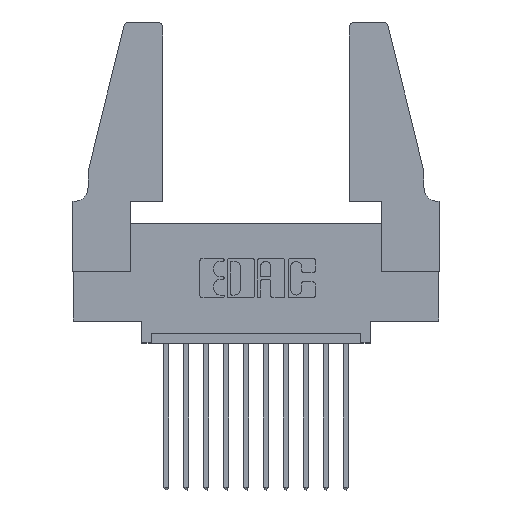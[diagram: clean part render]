
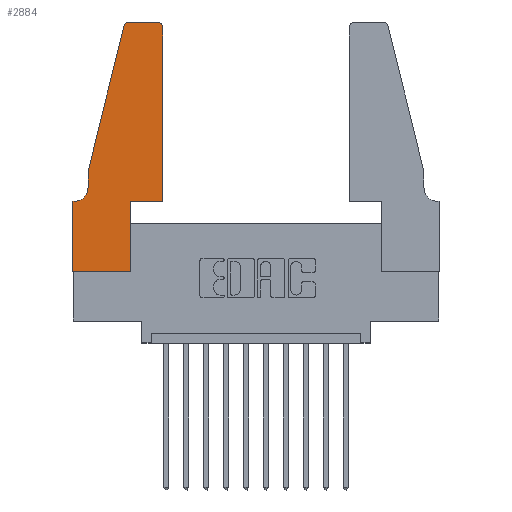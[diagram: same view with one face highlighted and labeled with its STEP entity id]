
A CAD part, top view. The second image highlights one B-rep face of the part: STEP entity #2884.
In plain terms, the highlighted planar face has unit normal (0, 0, 1).
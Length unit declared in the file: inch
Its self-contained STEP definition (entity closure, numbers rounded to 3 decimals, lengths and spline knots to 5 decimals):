
#29 = CARTESIAN_POINT ( 'NONE',  ( 0.2865, 0.35, 0.37 ) ) ;
#145 = LINE ( 'NONE', #1771, #10566 ) ;
#264 = VECTOR ( 'NONE', #11475, 39.37008 ) ;
#322 = AXIS2_PLACEMENT_3D ( 'NONE', #8340, #4215, #11858 ) ;
#350 = EDGE_CURVE ( 'NONE', #7436, #12567, #10413, .T. ) ;
#543 = ORIENTED_EDGE ( 'NONE', *, *, #13548, .T. ) ;
#614 = CARTESIAN_POINT ( 'NONE',  ( 0.2865, 0.35, 0.37 ) ) ;
#729 = LINE ( 'NONE', #6120, #3110 ) ;
#844 = VECTOR ( 'NONE', #7681, 39.37008 ) ;
#951 = VECTOR ( 'NONE', #7058, 39.37008 ) ;
#1074 = EDGE_CURVE ( 'NONE', #11638, #10250, #145, .T. ) ;
#1197 = ORIENTED_EDGE ( 'NONE', *, *, #11548, .T. ) ;
#1418 = VERTEX_POINT ( 'NONE', #29 ) ;
#1538 = VERTEX_POINT ( 'NONE', #4657 ) ;
#1735 = DIRECTION ( 'NONE',  ( 0., 0., -1. ) ) ;
#1771 = CARTESIAN_POINT ( 'NONE',  ( 0., 0., 0.37 ) ) ;
#1780 = LINE ( 'NONE', #6928, #264 ) ;
#2052 = EDGE_LOOP ( 'NONE', ( #7358, #9574, #12502, #6015, #12945, #13895, #11862, #543, #1197, #10156, #3249, #10666 ) ) ;
#2091 = CARTESIAN_POINT ( 'NONE',  ( 0., 0., 0.37 ) ) ;
#2102 = LINE ( 'NONE', #614, #4160 ) ;
#2114 = CIRCLE ( 'NONE', #3457, 0.03 ) ;
#2884 = ADVANCED_FACE ( 'NONE', ( #6073 ), #10430, .T. ) ;
#3110 = VECTOR ( 'NONE', #7028, 39.37008 ) ;
#3249 = ORIENTED_EDGE ( 'NONE', *, *, #4738, .T. ) ;
#3317 = CARTESIAN_POINT ( 'NONE',  ( 0.0755, 0.35, 0.37 ) ) ;
#3360 = VERTEX_POINT ( 'NONE', #12187 ) ;
#3457 = AXIS2_PLACEMENT_3D ( 'NONE', #10304, #4870, #12316 ) ;
#3508 = EDGE_CURVE ( 'NONE', #1418, #3654, #8292, .T. ) ;
#3521 = CARTESIAN_POINT ( 'NONE',  ( 0.284, 1.25, 0.37 ) ) ;
#3654 = VERTEX_POINT ( 'NONE', #13065 ) ;
#3735 = EDGE_CURVE ( 'NONE', #12781, #3360, #6061, .T. ) ;
#3913 = CARTESIAN_POINT ( 'NONE',  ( 0.4505, 0.35, 0.37 ) ) ;
#4008 = DIRECTION ( 'NONE',  ( 1., 0., 0. ) ) ;
#4160 = VECTOR ( 'NONE', #13800, 39.37008 ) ;
#4215 = DIRECTION ( 'NONE',  ( 0., 0., 1. ) ) ;
#4657 = CARTESIAN_POINT ( 'NONE',  ( 0.2865, 0., 0.37 ) ) ;
#4738 = EDGE_CURVE ( 'NONE', #3654, #9921, #729, .T. ) ;
#4870 = DIRECTION ( 'NONE',  ( 0., 0., 1. ) ) ;
#4915 = CARTESIAN_POINT ( 'NONE',  ( 0.0755, 0.5, 0.37 ) ) ;
#5088 = VERTEX_POINT ( 'NONE', #8239 ) ;
#5099 = CARTESIAN_POINT ( 'NONE',  ( 0.4505, 1.22, 0.37 ) ) ;
#5734 = LINE ( 'NONE', #3317, #11729 ) ;
#5951 = DIRECTION ( 'NONE',  ( 0., 0., 1. ) ) ;
#5979 = DIRECTION ( 'NONE',  ( -1., 0., 0. ) ) ;
#6015 = ORIENTED_EDGE ( 'NONE', *, *, #9546, .T. ) ;
#6061 = CIRCLE ( 'NONE', #7648, 0.07 ) ;
#6073 = FACE_OUTER_BOUND ( 'NONE', #2052, .T. ) ;
#6120 = CARTESIAN_POINT ( 'NONE',  ( 0.4505, 0.35, 0.37 ) ) ;
#6133 = AXIS2_PLACEMENT_3D ( 'NONE', #8189, #5951, #6865 ) ;
#6649 = LINE ( 'NONE', #10768, #844 ) ;
#6865 = DIRECTION ( 'NONE',  ( 1., 0., 0. ) ) ;
#6928 = CARTESIAN_POINT ( 'NONE',  ( 0.0755, 0.5, 0.37 ) ) ;
#7028 = DIRECTION ( 'NONE',  ( 0., 1., 0. ) ) ;
#7058 = DIRECTION ( 'NONE',  ( 0., -1., 0. ) ) ;
#7194 = CARTESIAN_POINT ( 'NONE',  ( 0.0055, 0.42, 0.37 ) ) ;
#7358 = ORIENTED_EDGE ( 'NONE', *, *, #350, .T. ) ;
#7436 = VERTEX_POINT ( 'NONE', #7452 ) ;
#7452 = CARTESIAN_POINT ( 'NONE',  ( 0.4205, 1.25, 0.37 ) ) ;
#7487 = CIRCLE ( 'NONE', #6133, 0.03 ) ;
#7648 = AXIS2_PLACEMENT_3D ( 'NONE', #7194, #1735, #12690 ) ;
#7681 = DIRECTION ( 'NONE',  ( 1., 0., 0. ) ) ;
#7960 = LINE ( 'NONE', #4915, #951 ) ;
#8189 = CARTESIAN_POINT ( 'NONE',  ( 0.284, 1.22, 0.37 ) ) ;
#8239 = CARTESIAN_POINT ( 'NONE',  ( 0.0755, 0.5, 0.37 ) ) ;
#8292 = LINE ( 'NONE', #3913, #10675 ) ;
#8305 = CARTESIAN_POINT ( 'NONE',  ( 0.0755, 0.42, 0.37 ) ) ;
#8340 = CARTESIAN_POINT ( 'NONE',  ( 0., 0.35, 0.37 ) ) ;
#8941 = EDGE_CURVE ( 'NONE', #11918, #5088, #1780, .T. ) ;
#9327 = EDGE_CURVE ( 'NONE', #12567, #11918, #7487, .T. ) ;
#9546 = EDGE_CURVE ( 'NONE', #5088, #12781, #7960, .T. ) ;
#9552 = VECTOR ( 'NONE', #5979, 39.37008 ) ;
#9574 = ORIENTED_EDGE ( 'NONE', *, *, #9327, .T. ) ;
#9765 = EDGE_CURVE ( 'NONE', #3360, #11638, #5734, .T. ) ;
#9921 = VERTEX_POINT ( 'NONE', #5099 ) ;
#9983 = CARTESIAN_POINT ( 'NONE',  ( 0.25487, 1.22718, 0.37 ) ) ;
#10156 = ORIENTED_EDGE ( 'NONE', *, *, #3508, .T. ) ;
#10250 = VERTEX_POINT ( 'NONE', #2091 ) ;
#10304 = CARTESIAN_POINT ( 'NONE',  ( 0.4205, 1.22, 0.37 ) ) ;
#10413 = LINE ( 'NONE', #12434, #9552 ) ;
#10430 = PLANE ( 'NONE',  #322 ) ;
#10566 = VECTOR ( 'NONE', #11637, 39.37008 ) ;
#10666 = ORIENTED_EDGE ( 'NONE', *, *, #11415, .T. ) ;
#10675 = VECTOR ( 'NONE', #4008, 39.37008 ) ;
#10768 = CARTESIAN_POINT ( 'NONE',  ( 0., 0., 0.37 ) ) ;
#11415 = EDGE_CURVE ( 'NONE', #9921, #7436, #2114, .T. ) ;
#11475 = DIRECTION ( 'NONE',  ( -0.239, -0.971, 0. ) ) ;
#11548 = EDGE_CURVE ( 'NONE', #1538, #1418, #2102, .T. ) ;
#11637 = DIRECTION ( 'NONE',  ( 0., -1., 0. ) ) ;
#11638 = VERTEX_POINT ( 'NONE', #12518 ) ;
#11729 = VECTOR ( 'NONE', #13019, 39.37008 ) ;
#11858 = DIRECTION ( 'NONE',  ( 1., 0., 0. ) ) ;
#11862 = ORIENTED_EDGE ( 'NONE', *, *, #1074, .T. ) ;
#11918 = VERTEX_POINT ( 'NONE', #9983 ) ;
#12187 = CARTESIAN_POINT ( 'NONE',  ( 0.0055, 0.35, 0.37 ) ) ;
#12316 = DIRECTION ( 'NONE',  ( 1., 0., 0. ) ) ;
#12434 = CARTESIAN_POINT ( 'NONE',  ( 0.2605, 1.25, 0.37 ) ) ;
#12502 = ORIENTED_EDGE ( 'NONE', *, *, #8941, .T. ) ;
#12518 = CARTESIAN_POINT ( 'NONE',  ( 0., 0.35, 0.37 ) ) ;
#12567 = VERTEX_POINT ( 'NONE', #3521 ) ;
#12690 = DIRECTION ( 'NONE',  ( -1., 0., 0. ) ) ;
#12781 = VERTEX_POINT ( 'NONE', #8305 ) ;
#12945 = ORIENTED_EDGE ( 'NONE', *, *, #3735, .T. ) ;
#13019 = DIRECTION ( 'NONE',  ( -1., 0., 0. ) ) ;
#13065 = CARTESIAN_POINT ( 'NONE',  ( 0.4505, 0.35, 0.37 ) ) ;
#13548 = EDGE_CURVE ( 'NONE', #10250, #1538, #6649, .T. ) ;
#13800 = DIRECTION ( 'NONE',  ( 0., 1., 0. ) ) ;
#13895 = ORIENTED_EDGE ( 'NONE', *, *, #9765, .T. ) ;
